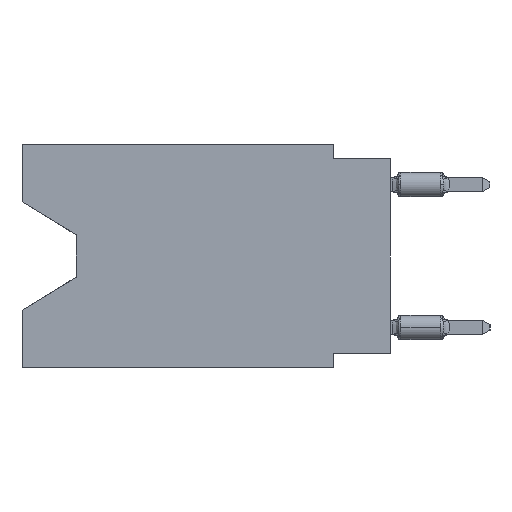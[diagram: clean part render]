
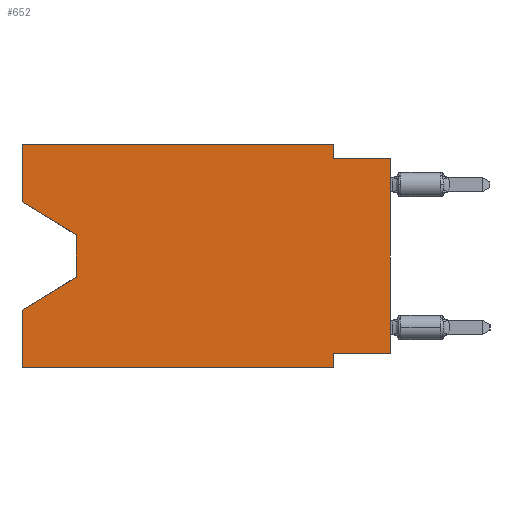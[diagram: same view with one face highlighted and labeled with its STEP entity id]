
A CAD part, left-side view. The second image highlights one B-rep face of the part: STEP entity #652.
In plain terms, the highlighted planar face has unit normal (-1, 0, 0).
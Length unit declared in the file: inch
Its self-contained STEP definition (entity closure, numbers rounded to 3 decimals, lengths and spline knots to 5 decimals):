
#168 = VERTEX_POINT ( 'NONE', #18130 ) ;
#652 = ADVANCED_FACE ( 'NONE', ( #24491 ), #18463, .F. ) ;
#791 = ORIENTED_EDGE ( 'NONE', *, *, #32254, .F. ) ;
#1188 = DIRECTION ( 'NONE',  ( 0., 0., -1. ) ) ;
#1503 = VERTEX_POINT ( 'NONE', #10219 ) ;
#1879 = EDGE_CURVE ( 'NONE', #1503, #20139, #18869, .T. ) ;
#1971 = EDGE_CURVE ( 'NONE', #19513, #1503, #10760, .T. ) ;
#2084 = EDGE_LOOP ( 'NONE', ( #30510, #29158, #17674, #16382, #24125, #25662, #21533, #24773, #38224, #791, #27511, #29347 ) ) ;
#2257 = VECTOR ( 'NONE', #20914, 39.37008 ) ;
#2534 = VECTOR ( 'NONE', #6353, 39.37008 ) ;
#2657 = EDGE_CURVE ( 'NONE', #33679, #168, #15037, .T. ) ;
#2683 = EDGE_CURVE ( 'NONE', #27380, #13943, #15633, .T. ) ;
#2941 = DIRECTION ( 'NONE',  ( 0., 0., 1. ) ) ;
#4413 = LINE ( 'NONE', #19919, #28535 ) ;
#4566 = VERTEX_POINT ( 'NONE', #8091 ) ;
#5573 = CARTESIAN_POINT ( 'NONE',  ( 0., 0., 0. ) ) ;
#5639 = CARTESIAN_POINT ( 'NONE',  ( 0., 0.55, -0.232 ) ) ;
#6353 = DIRECTION ( 'NONE',  ( 0., -1., 0. ) ) ;
#6952 = CARTESIAN_POINT ( 'NONE',  ( 0., 0.645, 0. ) ) ;
#7028 = VECTOR ( 'NONE', #2941, 39.37008 ) ;
#7791 = CARTESIAN_POINT ( 'NONE',  ( 0., 0.645, -0.10025 ) ) ;
#8091 = CARTESIAN_POINT ( 'NONE',  ( 0., 0.645, -0.28975 ) ) ;
#8800 = CARTESIAN_POINT ( 'NONE',  ( 0., 0., -0.365 ) ) ;
#9833 = EDGE_CURVE ( 'NONE', #19513, #22237, #20425, .T. ) ;
#10219 = CARTESIAN_POINT ( 'NONE',  ( 0., 0.645, 0. ) ) ;
#10372 = LINE ( 'NONE', #28914, #29278 ) ;
#10691 = EDGE_CURVE ( 'NONE', #27380, #37383, #20509, .T. ) ;
#10760 = LINE ( 'NONE', #6952, #30153 ) ;
#12232 = CARTESIAN_POINT ( 'NONE',  ( 0., 0.1, -0.365 ) ) ;
#13365 = CARTESIAN_POINT ( 'NONE',  ( 0., 0.645, -0.39 ) ) ;
#13943 = VERTEX_POINT ( 'NONE', #38140 ) ;
#14972 = CARTESIAN_POINT ( 'NONE',  ( 0., 0.55, -0.158 ) ) ;
#15037 = LINE ( 'NONE', #24676, #2534 ) ;
#15084 = CARTESIAN_POINT ( 'NONE',  ( 0., 0., -0.025 ) ) ;
#15633 = LINE ( 'NONE', #5573, #7028 ) ;
#16382 = ORIENTED_EDGE ( 'NONE', *, *, #29800, .F. ) ;
#17674 = ORIENTED_EDGE ( 'NONE', *, *, #39434, .T. ) ;
#18130 = CARTESIAN_POINT ( 'NONE',  ( 0., 0.1, -0.39 ) ) ;
#18463 = PLANE ( 'NONE',  #24816 ) ;
#18869 = LINE ( 'NONE', #37188, #37870 ) ;
#19513 = VERTEX_POINT ( 'NONE', #7791 ) ;
#19896 = DIRECTION ( 'NONE',  ( 0., 0., -1. ) ) ;
#19919 = CARTESIAN_POINT ( 'NONE',  ( 0., 0.1, -0.39 ) ) ;
#20139 = VERTEX_POINT ( 'NONE', #30488 ) ;
#20425 = LINE ( 'NONE', #35126, #37765 ) ;
#20509 = LINE ( 'NONE', #8800, #2257 ) ;
#20914 = DIRECTION ( 'NONE',  ( 0., 1., 0. ) ) ;
#21533 = ORIENTED_EDGE ( 'NONE', *, *, #10691, .F. ) ;
#22237 = VERTEX_POINT ( 'NONE', #14972 ) ;
#22894 = EDGE_CURVE ( 'NONE', #37383, #168, #4413, .T. ) ;
#23187 = DIRECTION ( 'NONE',  ( 0., -1., 0. ) ) ;
#23383 = LINE ( 'NONE', #15084, #37415 ) ;
#23621 = CARTESIAN_POINT ( 'NONE',  ( 0., 0.1, -0.025 ) ) ;
#24125 = ORIENTED_EDGE ( 'NONE', *, *, #2657, .T. ) ;
#24491 = FACE_OUTER_BOUND ( 'NONE', #2084, .T. ) ;
#24569 = LINE ( 'NONE', #33829, #38689 ) ;
#24676 = CARTESIAN_POINT ( 'NONE',  ( 0., 0.645, -0.39 ) ) ;
#24773 = ORIENTED_EDGE ( 'NONE', *, *, #2683, .T. ) ;
#24816 = AXIS2_PLACEMENT_3D ( 'NONE', #30542, #36584, #31128 ) ;
#25457 = EDGE_CURVE ( 'NONE', #38821, #13943, #23383, .T. ) ;
#25662 = ORIENTED_EDGE ( 'NONE', *, *, #22894, .F. ) ;
#25879 = DIRECTION ( 'NONE',  ( 0., 0., 1. ) ) ;
#26036 = DIRECTION ( 'NONE',  ( 0., -0.855, -0.519 ) ) ;
#26297 = VECTOR ( 'NONE', #19896, 39.37008 ) ;
#27380 = VERTEX_POINT ( 'NONE', #38947 ) ;
#27511 = ORIENTED_EDGE ( 'NONE', *, *, #1879, .F. ) ;
#28535 = VECTOR ( 'NONE', #1188, 39.37008 ) ;
#28914 = CARTESIAN_POINT ( 'NONE',  ( 0., 0.645, 0. ) ) ;
#28962 = CARTESIAN_POINT ( 'NONE',  ( 0., 0.55, -0.158 ) ) ;
#29158 = ORIENTED_EDGE ( 'NONE', *, *, #34858, .T. ) ;
#29278 = VECTOR ( 'NONE', #25879, 39.37008 ) ;
#29347 = ORIENTED_EDGE ( 'NONE', *, *, #1971, .F. ) ;
#29730 = LINE ( 'NONE', #38764, #37737 ) ;
#29800 = EDGE_CURVE ( 'NONE', #33679, #4566, #10372, .T. ) ;
#30153 = VECTOR ( 'NONE', #38166, 39.37008 ) ;
#30241 = VERTEX_POINT ( 'NONE', #5639 ) ;
#30488 = CARTESIAN_POINT ( 'NONE',  ( 0., 0.1, 0. ) ) ;
#30510 = ORIENTED_EDGE ( 'NONE', *, *, #9833, .T. ) ;
#30542 = CARTESIAN_POINT ( 'NONE',  ( 0., 0.645, 0. ) ) ;
#30814 = DIRECTION ( 'NONE',  ( 0., 0.855, -0.519 ) ) ;
#31128 = DIRECTION ( 'NONE',  ( 0., 0., -1. ) ) ;
#31978 = LINE ( 'NONE', #28962, #26297 ) ;
#32254 = EDGE_CURVE ( 'NONE', #20139, #38821, #29730, .T. ) ;
#32721 = DIRECTION ( 'NONE',  ( 0., 0., -1. ) ) ;
#33679 = VERTEX_POINT ( 'NONE', #13365 ) ;
#33829 = CARTESIAN_POINT ( 'NONE',  ( 0., 0.55, -0.232 ) ) ;
#34858 = EDGE_CURVE ( 'NONE', #22237, #30241, #31978, .T. ) ;
#35126 = CARTESIAN_POINT ( 'NONE',  ( 0., 0.645, -0.10025 ) ) ;
#36584 = DIRECTION ( 'NONE',  ( 1., 0., 0. ) ) ;
#37188 = CARTESIAN_POINT ( 'NONE',  ( 0., 0.645, 0. ) ) ;
#37377 = DIRECTION ( 'NONE',  ( 0., -1., 0. ) ) ;
#37383 = VERTEX_POINT ( 'NONE', #12232 ) ;
#37415 = VECTOR ( 'NONE', #23187, 39.37008 ) ;
#37737 = VECTOR ( 'NONE', #32721, 39.37008 ) ;
#37765 = VECTOR ( 'NONE', #26036, 39.37008 ) ;
#37870 = VECTOR ( 'NONE', #37377, 39.37008 ) ;
#38140 = CARTESIAN_POINT ( 'NONE',  ( 0., 0., -0.025 ) ) ;
#38166 = DIRECTION ( 'NONE',  ( 0., 0., 1. ) ) ;
#38224 = ORIENTED_EDGE ( 'NONE', *, *, #25457, .F. ) ;
#38689 = VECTOR ( 'NONE', #30814, 39.37008 ) ;
#38764 = CARTESIAN_POINT ( 'NONE',  ( 0., 0.1, 0. ) ) ;
#38821 = VERTEX_POINT ( 'NONE', #23621 ) ;
#38947 = CARTESIAN_POINT ( 'NONE',  ( 0., 0., -0.365 ) ) ;
#39434 = EDGE_CURVE ( 'NONE', #30241, #4566, #24569, .T. ) ;
